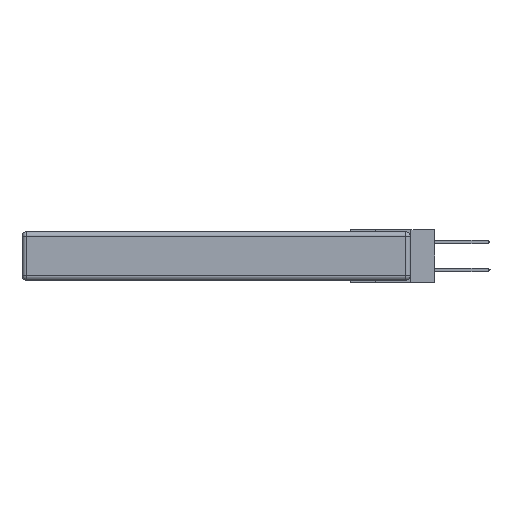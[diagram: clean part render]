
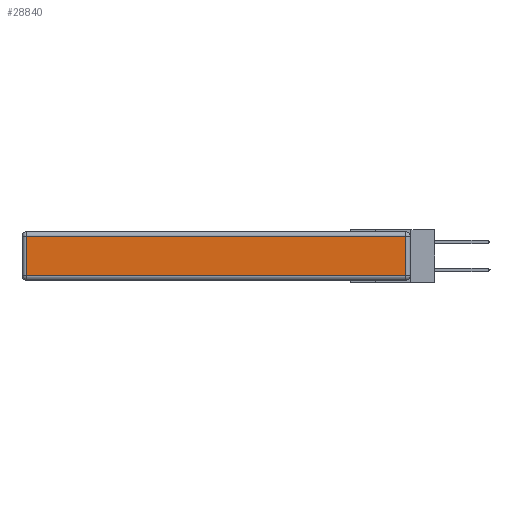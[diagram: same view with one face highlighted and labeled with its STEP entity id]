
A CAD part, left-side view. The second image highlights one B-rep face of the part: STEP entity #28840.
In plain terms, the highlighted planar face has unit normal (-1, 0, 0).
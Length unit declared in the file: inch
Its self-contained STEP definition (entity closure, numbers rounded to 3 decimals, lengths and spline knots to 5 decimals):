
#276 = DIRECTION ( 'NONE',  ( 0., 0., -1. ) ) ;
#1019 = LINE ( 'NONE', #20844, #18348 ) ;
#1357 = DIRECTION ( 'NONE',  ( -1., 0., 0. ) ) ;
#5270 = FACE_OUTER_BOUND ( 'NONE', #7342, .T. ) ;
#6215 = CARTESIAN_POINT ( 'NONE',  ( 0., 0.03, -0.03 ) ) ;
#6407 = ORIENTED_EDGE ( 'NONE', *, *, #10827, .T. ) ;
#6862 = EDGE_CURVE ( 'NONE', #24494, #19232, #31604, .T. ) ;
#7342 = EDGE_LOOP ( 'NONE', ( #10949, #23615, #25131, #6407 ) ) ;
#8788 = AXIS2_PLACEMENT_3D ( 'NONE', #30248, #1357, #22534 ) ;
#9526 = VERTEX_POINT ( 'NONE', #17742 ) ;
#9954 = DIRECTION ( 'NONE',  ( 0., 0., 1. ) ) ;
#10827 = EDGE_CURVE ( 'NONE', #19232, #9526, #1019, .T. ) ;
#10949 = ORIENTED_EDGE ( 'NONE', *, *, #27484, .T. ) ;
#11822 = VERTEX_POINT ( 'NONE', #32042 ) ;
#11873 = VECTOR ( 'NONE', #23526, 39.37008 ) ;
#12043 = PLANE ( 'NONE',  #8788 ) ;
#12761 = CARTESIAN_POINT ( 'NONE',  ( 0., 2.75, -0.03 ) ) ;
#16225 = LINE ( 'NONE', #25785, #29530 ) ;
#17531 = EDGE_CURVE ( 'NONE', #11822, #24494, #16225, .T. ) ;
#17742 = CARTESIAN_POINT ( 'NONE',  ( 0., 2.72, -0.313 ) ) ;
#18348 = VECTOR ( 'NONE', #276, 39.37008 ) ;
#19232 = VERTEX_POINT ( 'NONE', #23445 ) ;
#20844 = CARTESIAN_POINT ( 'NONE',  ( 0., 2.72, -0.343 ) ) ;
#22534 = DIRECTION ( 'NONE',  ( 0., 0., 1. ) ) ;
#22564 = VECTOR ( 'NONE', #25293, 39.37008 ) ;
#23445 = CARTESIAN_POINT ( 'NONE',  ( 0., 2.72, -0.03 ) ) ;
#23526 = DIRECTION ( 'NONE',  ( 0., -1., 0. ) ) ;
#23615 = ORIENTED_EDGE ( 'NONE', *, *, #17531, .T. ) ;
#24494 = VERTEX_POINT ( 'NONE', #6215 ) ;
#25131 = ORIENTED_EDGE ( 'NONE', *, *, #6862, .T. ) ;
#25293 = DIRECTION ( 'NONE',  ( 0., 1., 0. ) ) ;
#25785 = CARTESIAN_POINT ( 'NONE',  ( 0., 0.03, -0.343 ) ) ;
#26177 = CARTESIAN_POINT ( 'NONE',  ( 0., 0., -0.313 ) ) ;
#27484 = EDGE_CURVE ( 'NONE', #9526, #11822, #28104, .T. ) ;
#28104 = LINE ( 'NONE', #26177, #11873 ) ;
#28840 = ADVANCED_FACE ( 'NONE', ( #5270 ), #12043, .T. ) ;
#29530 = VECTOR ( 'NONE', #9954, 39.37008 ) ;
#30248 = CARTESIAN_POINT ( 'NONE',  ( 0., 0., -0.343 ) ) ;
#31604 = LINE ( 'NONE', #12761, #22564 ) ;
#32042 = CARTESIAN_POINT ( 'NONE',  ( 0., 0.03, -0.313 ) ) ;
